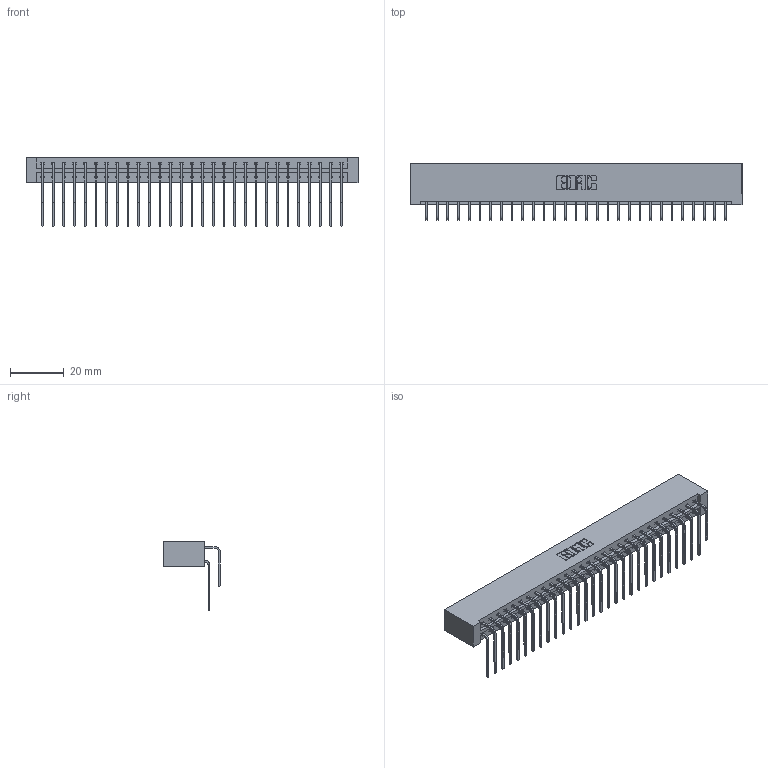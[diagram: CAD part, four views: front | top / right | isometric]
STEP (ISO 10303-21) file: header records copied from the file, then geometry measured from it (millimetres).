
FILE_DESCRIPTION (( 'STEP AP203' ), '1' );
FILE_NAME ('333-058-559-201.STEP', '2018-08-04T06:31:50', ( '' ), ( '' ), 'SwSTEP 2.0', 'SolidWorks 2016', '' );
FILE_SCHEMA (( 'CONFIG_CONTROL_DESIGN' ));
Length unit declared in the file: inch
Products named in the file (4): 333 Part_Lugless; 345-292-001_558 559 Tail - 1; 345-292-001_559 Tail - 2; 333-058-559-201
Assembly tree (59 placements, depth 2):
  333-058-559-201
    333 Part_Lugless
    345-292-001_558 559 Tail - 1  x29
    345-292-001_559 Tail - 2  x29
Bounding box: 123.16 x 20.9 x 25.53 mm (x, y, z)
Volume: 13419.6 mm3; surface area: 17416.6 mm2
Topology: 59 solids, 59 shells, 3238 faces, 9625 edges, 6338 vertices
Faces by surface type: plane 2270, cylinder 968
Entity records: 21845 total; most frequent: CARTESIAN_POINT 3685, ORIENTED_EDGE 3570, DIRECTION 3145, EDGE_CURVE 1785, VECTOR 1625, LINE 1625, VERTEX_POINT 1186, AXIS2_PLACEMENT_3D 760
